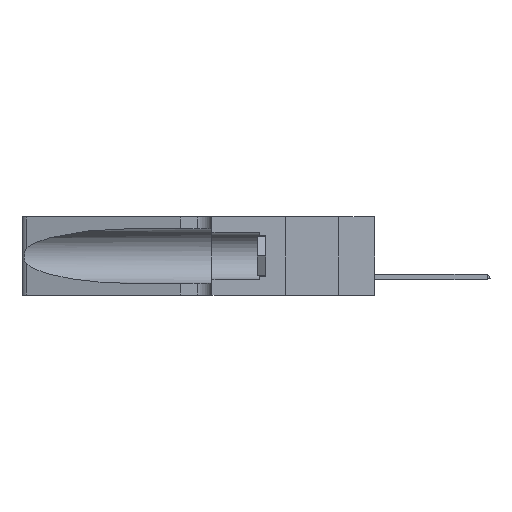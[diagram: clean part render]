
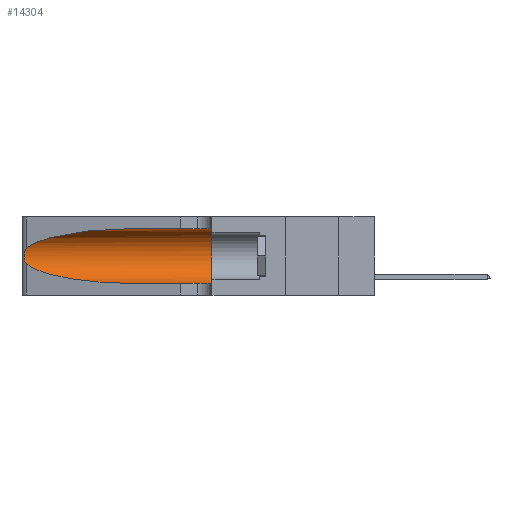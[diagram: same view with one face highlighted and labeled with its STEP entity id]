
A CAD part, left-side view. The second image highlights one B-rep face of the part: STEP entity #14304.
In plain terms, the highlighted cylindrical face has radius 3.308 mm (diameter 6.617 mm), a partial arc.
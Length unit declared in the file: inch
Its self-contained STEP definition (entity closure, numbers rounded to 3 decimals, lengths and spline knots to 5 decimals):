
#154 = EDGE_CURVE ( 'NONE', #20950, #16092, #25636, .T. ) ;
#556 = CYLINDRICAL_SURFACE ( 'NONE', #2430, 0.13025 ) ;
#733 = CARTESIAN_POINT ( 'NONE',  ( 0.1305, 0.72297, 0.05475 ) ) ;
#820 = VERTEX_POINT ( 'NONE', #4018 ) ;
#1607 = CARTESIAN_POINT ( 'NONE',  ( 0.1305, 0.72297, 0.31525 ) ) ;
#2371 = CARTESIAN_POINT ( 'NONE',  ( 0.1305, 0.35, 0.05475 ) ) ;
#2430 = AXIS2_PLACEMENT_3D ( 'NONE', #19505, #16493, #36126 ) ;
#2746 = CARTESIAN_POINT ( 'NONE',  ( 0.25487, 1.22718, 0.22369 ) ) ;
#2876 = B_SPLINE_CURVE_WITH_KNOTS ( 'NONE', 3,
 ( #25971, #20572, #31592, #6285, #23478, #17312, #20080, #11842, #3488, #17560, #9163, #5899, #6414, #25850 ),
 .UNSPECIFIED., .F., .F.,
 ( 4, 2, 2, 2, 2, 2, 4 ),
 ( 0., 0.00027, 0.00053, 0.00107, 0.0016, 0.00187, 0.00214 ),
 .UNSPECIFIED. ) ;
#3488 = CARTESIAN_POINT ( 'NONE',  ( 0.26017, 1.23833, 0.17102 ) ) ;
#3687 = EDGE_CURVE ( 'NONE', #820, #20049, #7385, .T. ) ;
#3762 = VECTOR ( 'NONE', #18518, 39.37008 ) ;
#4018 = CARTESIAN_POINT ( 'NONE',  ( 0.1305, 0.72297, 0.05475 ) ) ;
#4563 = ORIENTED_EDGE ( 'NONE', *, *, #154, .F. ) ;
#5483 = DIRECTION ( 'NONE',  ( 0., 0., 1. ) ) ;
#5899 = CARTESIAN_POINT ( 'NONE',  ( 0.25639, 1.23186, 0.15144 ) ) ;
#6285 = CARTESIAN_POINT ( 'NONE',  ( 0.25787, 1.23484, 0.2124 ) ) ;
#6414 = CARTESIAN_POINT ( 'NONE',  ( 0.25555, 1.22993, 0.14849 ) ) ;
#6563 = AXIS2_PLACEMENT_3D ( 'NONE', #16403, #36409, #5483 ) ;
#7385 = LINE ( 'NONE', #24451, #3762 ) ;
#9163 = CARTESIAN_POINT ( 'NONE',  ( 0.25789, 1.23486, 0.15765 ) ) ;
#10100 = ORIENTED_EDGE ( 'NONE', *, *, #29355, .F. ) ;
#11842 = CARTESIAN_POINT ( 'NONE',  ( 0.26075, 1.23896, 0.178 ) ) ;
#11869 = VERTEX_POINT ( 'NONE', #21112 ) ;
#12247 = CARTESIAN_POINT ( 'NONE',  ( 0.1305, 1.61858, 0.31525 ) ) ;
#13293 = ORIENTED_EDGE ( 'NONE', *, *, #27023, .T. ) ;
#14304 = ADVANCED_FACE ( 'NONE', ( #30434 ), #556, .F. ) ;
#14447 = CARTESIAN_POINT ( 'NONE',  ( 0.18966, 0.96281, 0.31525 ) ) ;
#15377 = EDGE_LOOP ( 'NONE', ( #13293, #20571, #29365, #31674, #10100, #4563 ) ) ;
#16092 = VERTEX_POINT ( 'NONE', #31681 ) ;
#16403 = CARTESIAN_POINT ( 'NONE',  ( 0.1305, 0.35, 0.185 ) ) ;
#16493 = DIRECTION ( 'NONE',  ( 0., -1., 0. ) ) ;
#17312 = CARTESIAN_POINT ( 'NONE',  ( 0.26018, 1.23835, 0.19895 ) ) ;
#17560 = CARTESIAN_POINT ( 'NONE',  ( 0.25856, 1.23593, 0.16098 ) ) ;
#18518 = DIRECTION ( 'NONE',  ( 0., -1., 0. ) ) ;
#19505 = CARTESIAN_POINT ( 'NONE',  ( 0.1305, 1.61858, 0.185 ) ) ;
#20049 = VERTEX_POINT ( 'NONE', #2371 ) ;
#20080 = CARTESIAN_POINT ( 'NONE',  ( 0.26075, 1.23896, 0.19203 ) ) ;
#20109 = EDGE_CURVE ( 'NONE', #31035, #11869, #2876, .T. ) ;
#20312 = CARTESIAN_POINT ( 'NONE',  ( 0.1305, 0.72297, 0.31525 ) ) ;
#20571 = ORIENTED_EDGE ( 'NONE', *, *, #20109, .T. ) ;
#20572 = CARTESIAN_POINT ( 'NONE',  ( 0.25555, 1.22994, 0.2215 ) ) ;
#20831 = CARTESIAN_POINT ( 'NONE',  ( 0.2373, 1.15595, 0.08982 ) ) ;
#20950 = VERTEX_POINT ( 'NONE', #1607 ) ;
#21112 = CARTESIAN_POINT ( 'NONE',  ( 0.25487, 1.22718, 0.14631 ) ) ;
#22317 =( BOUNDED_CURVE ( )  B_SPLINE_CURVE ( 3, ( #20312, #14447, #25966, #2746 ),
 .UNSPECIFIED., .F., .F. ) 
 B_SPLINE_CURVE_WITH_KNOTS ( ( 4, 4 ),
 ( 1.5708, 2.84003 ),
 .UNSPECIFIED. ) 
 CURVE ( )  GEOMETRIC_REPRESENTATION_ITEM ( )  RATIONAL_B_SPLINE_CURVE ( ( 1., 0.87, 0.87, 1. ) ) 
 REPRESENTATION_ITEM ( '' )  );
#23478 = CARTESIAN_POINT ( 'NONE',  ( 0.25854, 1.2359, 0.20912 ) ) ;
#24451 = CARTESIAN_POINT ( 'NONE',  ( 0.1305, 1.61858, 0.05475 ) ) ;
#24715 = VECTOR ( 'NONE', #26627, 39.37008 ) ;
#25636 = LINE ( 'NONE', #12247, #24715 ) ;
#25850 = CARTESIAN_POINT ( 'NONE',  ( 0.25487, 1.22718, 0.14631 ) ) ;
#25966 = CARTESIAN_POINT ( 'NONE',  ( 0.2373, 1.15595, 0.28018 ) ) ;
#25971 = CARTESIAN_POINT ( 'NONE',  ( 0.25487, 1.22718, 0.22369 ) ) ;
#26627 = DIRECTION ( 'NONE',  ( 0., -1., 0. ) ) ;
#26675 =( BOUNDED_CURVE ( )  B_SPLINE_CURVE ( 3, ( #32207, #20831, #28982, #733 ),
 .UNSPECIFIED., .F., .F. ) 
 B_SPLINE_CURVE_WITH_KNOTS ( ( 4, 4 ),
 ( 3.44316, 4.71239 ),
 .UNSPECIFIED. ) 
 CURVE ( )  GEOMETRIC_REPRESENTATION_ITEM ( )  RATIONAL_B_SPLINE_CURVE ( ( 1., 0.87, 0.87, 1. ) ) 
 REPRESENTATION_ITEM ( '' )  );
#27023 = EDGE_CURVE ( 'NONE', #20950, #31035, #22317, .T. ) ;
#28858 = CARTESIAN_POINT ( 'NONE',  ( 0.25487, 1.22718, 0.22369 ) ) ;
#28982 = CARTESIAN_POINT ( 'NONE',  ( 0.18966, 0.96281, 0.05475 ) ) ;
#29355 = EDGE_CURVE ( 'NONE', #16092, #20049, #32449, .T. ) ;
#29365 = ORIENTED_EDGE ( 'NONE', *, *, #34599, .T. ) ;
#30434 = FACE_OUTER_BOUND ( 'NONE', #15377, .T. ) ;
#31035 = VERTEX_POINT ( 'NONE', #28858 ) ;
#31592 = CARTESIAN_POINT ( 'NONE',  ( 0.25639, 1.23184, 0.21858 ) ) ;
#31674 = ORIENTED_EDGE ( 'NONE', *, *, #3687, .T. ) ;
#31681 = CARTESIAN_POINT ( 'NONE',  ( 0.1305, 0.35, 0.31525 ) ) ;
#32207 = CARTESIAN_POINT ( 'NONE',  ( 0.25487, 1.22718, 0.14631 ) ) ;
#32449 = CIRCLE ( 'NONE', #6563, 0.13025 ) ;
#34599 = EDGE_CURVE ( 'NONE', #11869, #820, #26675, .T. ) ;
#36126 = DIRECTION ( 'NONE',  ( 0., 0., -1. ) ) ;
#36409 = DIRECTION ( 'NONE',  ( 0., 1., 0. ) ) ;
